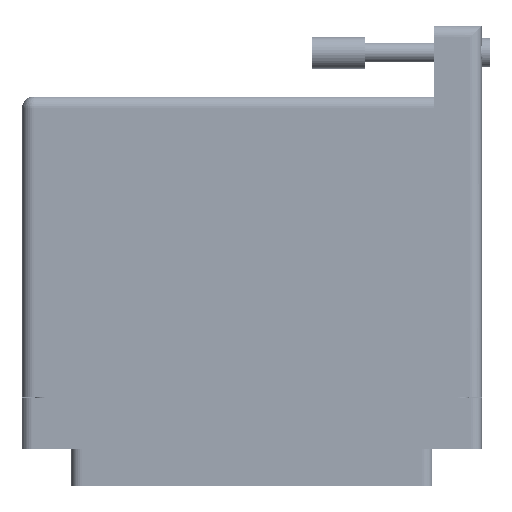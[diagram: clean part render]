
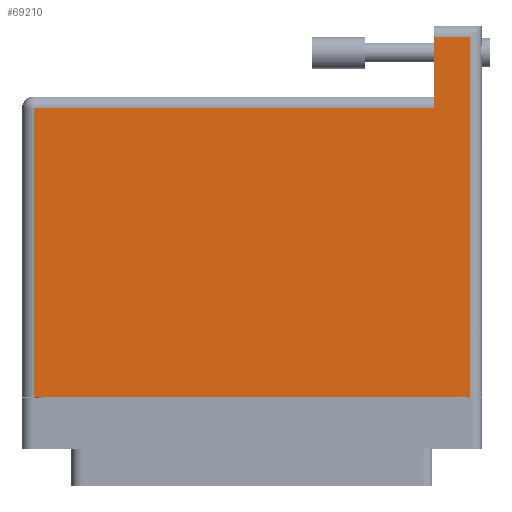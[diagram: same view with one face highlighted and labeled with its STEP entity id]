
A CAD part, front view. The second image highlights one B-rep face of the part: STEP entity #69210.
In plain terms, the highlighted face is planar.
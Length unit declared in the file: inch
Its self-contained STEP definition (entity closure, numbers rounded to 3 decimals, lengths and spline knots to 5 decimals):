
#274 = VERTEX_POINT ( 'NONE', #14230 ) ;
#7551 = VECTOR ( 'NONE', #59372, 39.37008 ) ;
#7934 = ORIENTED_EDGE ( 'NONE', *, *, #17889, .T. ) ;
#8990 = ORIENTED_EDGE ( 'NONE', *, *, #63307, .T. ) ;
#10662 = DIRECTION ( 'NONE',  ( -1., 0., 0. ) ) ;
#12073 = VERTEX_POINT ( 'NONE', #38548 ) ;
#14185 = VECTOR ( 'NONE', #53742, 39.37008 ) ;
#14230 = CARTESIAN_POINT ( 'NONE',  ( 1.079, 2.025, 0.617 ) ) ;
#16513 = VERTEX_POINT ( 'NONE', #33312 ) ;
#17889 = EDGE_CURVE ( 'NONE', #274, #37013, #54124, .T. ) ;
#17986 = ORIENTED_EDGE ( 'NONE', *, *, #18157, .T. ) ;
#18157 = EDGE_CURVE ( 'NONE', #16513, #35285, #62620, .T. ) ;
#20885 = CARTESIAN_POINT ( 'NONE',  ( -1.359, 2.025, 0.617 ) ) ;
#21375 = DIRECTION ( 'NONE',  ( 0., -1., 0. ) ) ;
#25340 = LINE ( 'NONE', #37633, #7551 ) ;
#26692 = LINE ( 'NONE', #35736, #33496 ) ;
#26811 = CARTESIAN_POINT ( 'NONE',  ( -1.359, 1.675, 0.617 ) ) ;
#27587 = CARTESIAN_POINT ( 'NONE',  ( 1.289, 2.025, 0.617 ) ) ;
#29310 = DIRECTION ( 'NONE',  ( 1., 0., 0. ) ) ;
#30288 = LINE ( 'NONE', #20885, #14185 ) ;
#31089 = DIRECTION ( 'NONE',  ( 0., 1., 0. ) ) ;
#32526 = EDGE_CURVE ( 'NONE', #61425, #12073, #49426, .T. ) ;
#32797 = ORIENTED_EDGE ( 'NONE', *, *, #40728, .T. ) ;
#33312 = CARTESIAN_POINT ( 'NONE',  ( 1.289, -0.1, 0.617 ) ) ;
#33496 = VECTOR ( 'NONE', #29310, 39.37008 ) ;
#35021 = EDGE_LOOP ( 'NONE', ( #32797, #56719, #8990, #17986, #39995, #7934 ) ) ;
#35074 = VECTOR ( 'NONE', #21375, 39.37008 ) ;
#35285 = VERTEX_POINT ( 'NONE', #27587 ) ;
#35366 = CARTESIAN_POINT ( 'NONE',  ( 1.289, 2.095, 0.617 ) ) ;
#35736 = CARTESIAN_POINT ( 'NONE',  ( -1.359, -0.1, 0.617 ) ) ;
#36428 = VECTOR ( 'NONE', #31089, 39.37008 ) ;
#37013 = VERTEX_POINT ( 'NONE', #50817 ) ;
#37633 = CARTESIAN_POINT ( 'NONE',  ( -1.359, 1.605, 0.617 ) ) ;
#37923 = PLANE ( 'NONE',  #66878 ) ;
#38508 = CARTESIAN_POINT ( 'NONE',  ( 1.079, 2.095, 0.617 ) ) ;
#38548 = CARTESIAN_POINT ( 'NONE',  ( -1.289, -0.1, 0.617 ) ) ;
#39995 = ORIENTED_EDGE ( 'NONE', *, *, #43596, .T. ) ;
#40728 = EDGE_CURVE ( 'NONE', #37013, #61425, #25340, .T. ) ;
#43596 = EDGE_CURVE ( 'NONE', #35285, #274, #30288, .T. ) ;
#48258 = VECTOR ( 'NONE', #49341, 39.37008 ) ;
#49341 = DIRECTION ( 'NONE',  ( 0., -1., 0. ) ) ;
#49426 = LINE ( 'NONE', #53537, #35074 ) ;
#50817 = CARTESIAN_POINT ( 'NONE',  ( 1.079, 1.605, 0.617 ) ) ;
#53537 = CARTESIAN_POINT ( 'NONE',  ( -1.289, -0.1, 0.617 ) ) ;
#53742 = DIRECTION ( 'NONE',  ( -1., 0., 0. ) ) ;
#54076 = FACE_OUTER_BOUND ( 'NONE', #35021, .T. ) ;
#54124 = LINE ( 'NONE', #38508, #48258 ) ;
#56470 = CARTESIAN_POINT ( 'NONE',  ( -1.289, 1.605, 0.617 ) ) ;
#56719 = ORIENTED_EDGE ( 'NONE', *, *, #32526, .T. ) ;
#59372 = DIRECTION ( 'NONE',  ( -1., 0., 0. ) ) ;
#61425 = VERTEX_POINT ( 'NONE', #56470 ) ;
#62620 = LINE ( 'NONE', #35366, #36428 ) ;
#63307 = EDGE_CURVE ( 'NONE', #12073, #16513, #26692, .T. ) ;
#64152 = DIRECTION ( 'NONE',  ( 0., 0., -1. ) ) ;
#66878 = AXIS2_PLACEMENT_3D ( 'NONE', #26811, #64152, #10662 ) ;
#69210 = ADVANCED_FACE ( 'NONE', ( #54076 ), #37923, .F. ) ;
